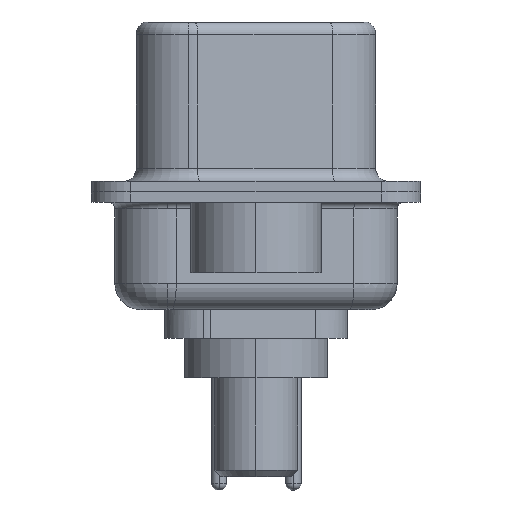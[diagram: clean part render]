
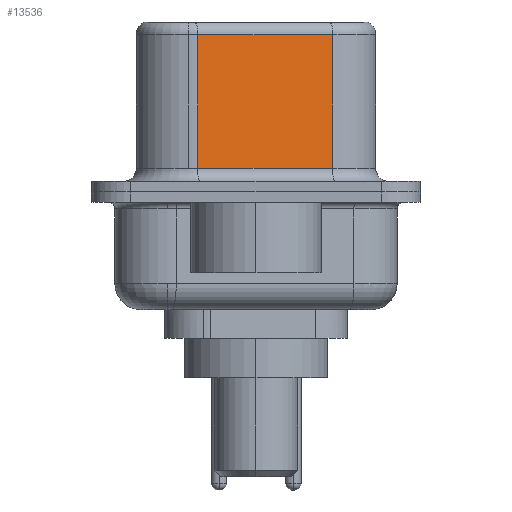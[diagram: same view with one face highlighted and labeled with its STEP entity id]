
A CAD part, left-side view. The second image highlights one B-rep face of the part: STEP entity #13536.
In plain terms, the highlighted planar face has unit normal (-0.985, -0.174, 0).
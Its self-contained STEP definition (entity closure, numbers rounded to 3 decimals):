
#1318 = EDGE_LOOP ( 'NONE', ( #11507, #1984, #12910, #8158 ) ) ;
#1473 = CARTESIAN_POINT ( 'NONE',  ( 4.585, -2.927, 6.52 ) ) ;
#1796 = VERTEX_POINT ( 'NONE', #6296 ) ;
#1984 = ORIENTED_EDGE ( 'NONE', *, *, #12123, .T. ) ;
#2316 = VECTOR ( 'NONE', #4281, 1000. ) ;
#2434 = CARTESIAN_POINT ( 'NONE',  ( 4.585, -2.927, 0.9 ) ) ;
#2502 = CARTESIAN_POINT ( 'NONE',  ( 3.675, 2.233, 6.02 ) ) ;
#2709 = VECTOR ( 'NONE', #5442, 1000. ) ;
#2900 = DIRECTION ( 'NONE',  ( -0.174, 0.985, 0. ) ) ;
#4281 = DIRECTION ( 'NONE',  ( -0.174, 0.985, 0. ) ) ;
#4300 = FACE_OUTER_BOUND ( 'NONE', #1318, .T. ) ;
#5233 = VERTEX_POINT ( 'NONE', #2502 ) ;
#5442 = DIRECTION ( 'NONE',  ( 0., 0., -1. ) ) ;
#5464 = EDGE_CURVE ( 'NONE', #1796, #9765, #11624, .T. ) ;
#6296 = CARTESIAN_POINT ( 'NONE',  ( 3.675, 2.233, 0.9 ) ) ;
#7136 = CARTESIAN_POINT ( 'NONE',  ( 4.585, -2.927, 6.02 ) ) ;
#7789 = VECTOR ( 'NONE', #8058, 1000. ) ;
#8058 = DIRECTION ( 'NONE',  ( 0., 0., -1. ) ) ;
#8158 = ORIENTED_EDGE ( 'NONE', *, *, #5464, .T. ) ;
#8507 = PLANE ( 'NONE',  #18037 ) ;
#8872 = CARTESIAN_POINT ( 'NONE',  ( 4.585, -2.927, 6.02 ) ) ;
#9744 = CARTESIAN_POINT ( 'NONE',  ( 3.675, 2.233, 6.52 ) ) ;
#9765 = VERTEX_POINT ( 'NONE', #14919 ) ;
#10515 = DIRECTION ( 'NONE',  ( 0.174, -0.985, 0. ) ) ;
#11098 = LINE ( 'NONE', #9744, #2709 ) ;
#11370 = DIRECTION ( 'NONE',  ( 0.985, 0.174, 0. ) ) ;
#11507 = ORIENTED_EDGE ( 'NONE', *, *, #14980, .F. ) ;
#11624 = LINE ( 'NONE', #2434, #14962 ) ;
#12123 = EDGE_CURVE ( 'NONE', #15292, #5233, #14049, .T. ) ;
#12910 = ORIENTED_EDGE ( 'NONE', *, *, #16292, .T. ) ;
#13536 = ADVANCED_FACE ( 'NONE', ( #4300 ), #8507, .F. ) ;
#14049 = LINE ( 'NONE', #7136, #2316 ) ;
#14919 = CARTESIAN_POINT ( 'NONE',  ( 4.585, -2.927, 0.9 ) ) ;
#14962 = VECTOR ( 'NONE', #10515, 1000. ) ;
#14980 = EDGE_CURVE ( 'NONE', #15292, #9765, #15343, .T. ) ;
#15292 = VERTEX_POINT ( 'NONE', #8872 ) ;
#15343 = LINE ( 'NONE', #17954, #7789 ) ;
#16292 = EDGE_CURVE ( 'NONE', #5233, #1796, #11098, .T. ) ;
#17954 = CARTESIAN_POINT ( 'NONE',  ( 4.585, -2.927, 6.52 ) ) ;
#18037 = AXIS2_PLACEMENT_3D ( 'NONE', #1473, #11370, #2900 ) ;
